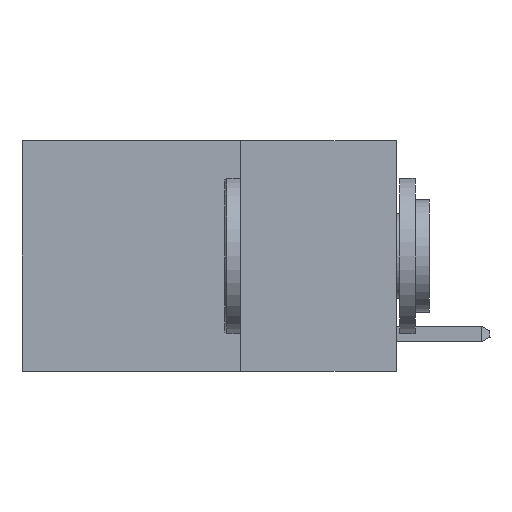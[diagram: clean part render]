
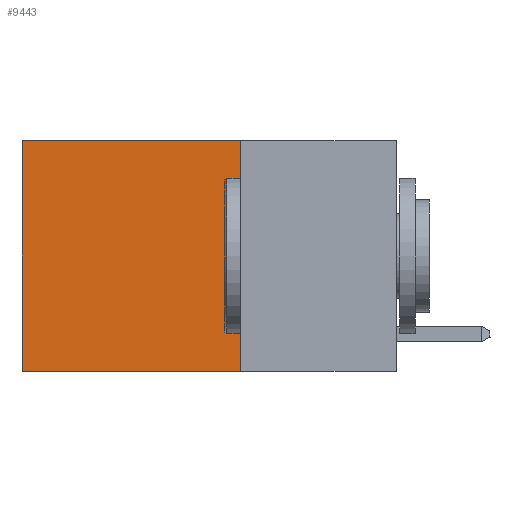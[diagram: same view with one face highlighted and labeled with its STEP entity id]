
A CAD part, left-side view. The second image highlights one B-rep face of the part: STEP entity #9443.
In plain terms, the highlighted planar face has unit normal (-1, 0, 0).
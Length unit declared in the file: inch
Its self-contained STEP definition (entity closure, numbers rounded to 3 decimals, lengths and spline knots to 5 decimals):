
#695 = CARTESIAN_POINT ( 'NONE',  ( 0.2625, 0.25, -0.37 ) ) ;
#809 = DIRECTION ( 'NONE',  ( 0., 1., 0. ) ) ;
#1239 = DIRECTION ( 'NONE',  ( 0., 0., -1. ) ) ;
#2044 = DIRECTION ( 'NONE',  ( 0., 1., 0. ) ) ;
#2120 = DIRECTION ( 'NONE',  ( 1., 0., 0. ) ) ;
#2905 = EDGE_CURVE ( 'NONE', #19002, #20219, #18569, .T. ) ;
#2965 = CARTESIAN_POINT ( 'NONE',  ( 0.2625, 0.6, -0.37 ) ) ;
#3445 = VERTEX_POINT ( 'NONE', #12267 ) ;
#3529 = PLANE ( 'NONE',  #18817 ) ;
#3530 = ORIENTED_EDGE ( 'NONE', *, *, #2905, .T. ) ;
#3754 = ORIENTED_EDGE ( 'NONE', *, *, #17665, .F. ) ;
#4421 = EDGE_LOOP ( 'NONE', ( #3530, #7058, #3754, #8472 ) ) ;
#4958 = VERTEX_POINT ( 'NONE', #6647 ) ;
#5028 = VECTOR ( 'NONE', #2044, 39.37008 ) ;
#6011 = EDGE_CURVE ( 'NONE', #4958, #19002, #8863, .T. ) ;
#6647 = CARTESIAN_POINT ( 'NONE',  ( 0.2625, 0.25, 0. ) ) ;
#7058 = ORIENTED_EDGE ( 'NONE', *, *, #11349, .F. ) ;
#7672 = VECTOR ( 'NONE', #13580, 39.37008 ) ;
#7936 = CARTESIAN_POINT ( 'NONE',  ( 0.2625, 0.25, 0. ) ) ;
#8472 = ORIENTED_EDGE ( 'NONE', *, *, #6011, .T. ) ;
#8863 = LINE ( 'NONE', #10492, #5028 ) ;
#9443 = ADVANCED_FACE ( 'NONE', ( #10132 ), #3529, .F. ) ;
#9887 = CARTESIAN_POINT ( 'NONE',  ( 0.2625, 0.6, 0. ) ) ;
#10132 = FACE_OUTER_BOUND ( 'NONE', #4421, .T. ) ;
#10492 = CARTESIAN_POINT ( 'NONE',  ( 0.2625, 0.25, 0. ) ) ;
#11349 = EDGE_CURVE ( 'NONE', #3445, #20219, #17457, .T. ) ;
#11873 = CARTESIAN_POINT ( 'NONE',  ( 0.2625, 0.25, 0. ) ) ;
#11883 = VECTOR ( 'NONE', #809, 39.37008 ) ;
#11979 = DIRECTION ( 'NONE',  ( 0., 0., -1. ) ) ;
#12267 = CARTESIAN_POINT ( 'NONE',  ( 0.2625, 0.25, -0.37 ) ) ;
#13477 = CARTESIAN_POINT ( 'NONE',  ( 0.2625, 0.6, 0. ) ) ;
#13580 = DIRECTION ( 'NONE',  ( 0., 0., -1. ) ) ;
#14477 = VECTOR ( 'NONE', #1239, 39.37008 ) ;
#16164 = LINE ( 'NONE', #7936, #14477 ) ;
#17457 = LINE ( 'NONE', #695, #11883 ) ;
#17665 = EDGE_CURVE ( 'NONE', #4958, #3445, #16164, .T. ) ;
#18569 = LINE ( 'NONE', #13477, #7672 ) ;
#18817 = AXIS2_PLACEMENT_3D ( 'NONE', #11873, #2120, #11979 ) ;
#19002 = VERTEX_POINT ( 'NONE', #9887 ) ;
#20219 = VERTEX_POINT ( 'NONE', #2965 ) ;
